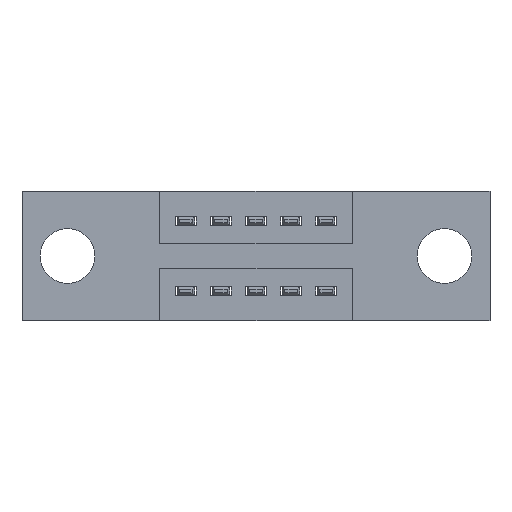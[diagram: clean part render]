
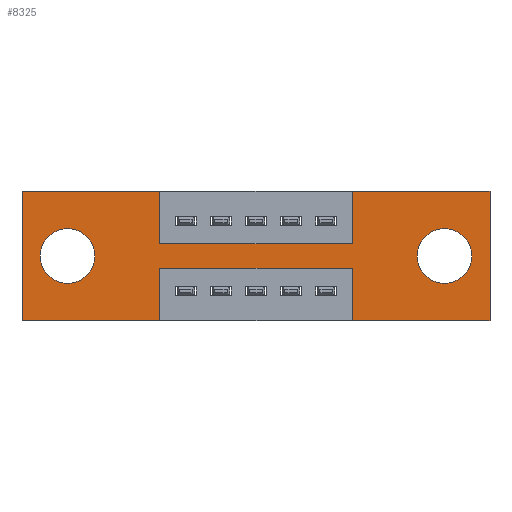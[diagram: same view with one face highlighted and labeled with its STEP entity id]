
A CAD part, front view. The second image highlights one B-rep face of the part: STEP entity #8325.
In plain terms, the highlighted planar face has unit normal (0, -1, 0).
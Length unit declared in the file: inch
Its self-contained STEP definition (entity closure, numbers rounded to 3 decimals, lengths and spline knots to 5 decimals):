
#27 = DIRECTION ( 'NONE',  ( 0., 0., -1. ) ) ;
#56 = CIRCLE ( 'NONE', #2619, 0.078 ) ;
#59 = CIRCLE ( 'NONE', #1636, 0.078 ) ;
#77 = EDGE_CURVE ( 'NONE', #8403, #8178, #6457, .T. ) ;
#88 = VECTOR ( 'NONE', #1015, 39.37008 ) ;
#94 = LINE ( 'NONE', #2735, #6843 ) ;
#206 = DIRECTION ( 'NONE',  ( 0., 0., -1. ) ) ;
#236 = EDGE_CURVE ( 'NONE', #5927, #4258, #5038, .T. ) ;
#280 = ORIENTED_EDGE ( 'NONE', *, *, #5245, .F. ) ;
#344 = EDGE_CURVE ( 'NONE', #1747, #5927, #2387, .T. ) ;
#406 = EDGE_CURVE ( 'NONE', #2341, #8580, #4386, .T. ) ;
#566 = DIRECTION ( 'NONE',  ( 0., 0., -1. ) ) ;
#583 = ORIENTED_EDGE ( 'NONE', *, *, #406, .F. ) ;
#667 = CARTESIAN_POINT ( 'NONE',  ( 0.3925, 0., -0.15 ) ) ;
#710 = PLANE ( 'NONE',  #906 ) ;
#735 = DIRECTION ( 'NONE',  ( 1., 0., 0. ) ) ;
#906 = AXIS2_PLACEMENT_3D ( 'NONE', #5362, #3974, #27 ) ;
#981 = CARTESIAN_POINT ( 'NONE',  ( 1.205, 0., -0.107 ) ) ;
#1015 = DIRECTION ( 'NONE',  ( -1., 0., 0. ) ) ;
#1120 = CARTESIAN_POINT ( 'NONE',  ( 0., 0., 0. ) ) ;
#1133 = CARTESIAN_POINT ( 'NONE',  ( 0., 0., 0. ) ) ;
#1135 = LINE ( 'NONE', #8387, #2388 ) ;
#1307 = ORIENTED_EDGE ( 'NONE', *, *, #236, .F. ) ;
#1377 = ORIENTED_EDGE ( 'NONE', *, *, #7110, .F. ) ;
#1396 = DIRECTION ( 'NONE',  ( -1., 0., 0. ) ) ;
#1445 = DIRECTION ( 'NONE',  ( 0., 1., 0. ) ) ;
#1485 = ORIENTED_EDGE ( 'NONE', *, *, #7705, .F. ) ;
#1506 = EDGE_CURVE ( 'NONE', #4596, #8403, #6110, .T. ) ;
#1546 = CARTESIAN_POINT ( 'NONE',  ( 0.3925, 0., -0.37 ) ) ;
#1636 = AXIS2_PLACEMENT_3D ( 'NONE', #3687, #2991, #3114 ) ;
#1641 = DIRECTION ( 'NONE',  ( 0., 0., 1. ) ) ;
#1666 = VERTEX_POINT ( 'NONE', #4613 ) ;
#1695 = EDGE_LOOP ( 'NONE', ( #1485, #3942, #583, #1377, #2358, #280, #1307, #4324, #3723, #8166, #3185, #7621 ) ) ;
#1747 = VERTEX_POINT ( 'NONE', #667 ) ;
#1890 = CARTESIAN_POINT ( 'NONE',  ( 0.9425, 0., 0. ) ) ;
#1973 = CARTESIAN_POINT ( 'NONE',  ( 0., 0., 0. ) ) ;
#2021 = CARTESIAN_POINT ( 'NONE',  ( 0., 0., -0.37 ) ) ;
#2030 = CARTESIAN_POINT ( 'NONE',  ( 0.9425, 0., -0.37 ) ) ;
#2341 = VERTEX_POINT ( 'NONE', #4839 ) ;
#2358 = ORIENTED_EDGE ( 'NONE', *, *, #3750, .F. ) ;
#2387 = LINE ( 'NONE', #4078, #6714 ) ;
#2388 = VECTOR ( 'NONE', #2389, 39.37008 ) ;
#2389 = DIRECTION ( 'NONE',  ( 1., 0., 0. ) ) ;
#2505 = EDGE_CURVE ( 'NONE', #8580, #6228, #8431, .T. ) ;
#2516 = VECTOR ( 'NONE', #1396, 39.37008 ) ;
#2595 = VECTOR ( 'NONE', #7276, 39.37008 ) ;
#2619 = AXIS2_PLACEMENT_3D ( 'NONE', #6319, #2947, #1641 ) ;
#2651 = ORIENTED_EDGE ( 'NONE', *, *, #5657, .T. ) ;
#2672 = ORIENTED_EDGE ( 'NONE', *, *, #6633, .T. ) ;
#2735 = CARTESIAN_POINT ( 'NONE',  ( 0., 0., -0.37 ) ) ;
#2790 = VECTOR ( 'NONE', #5843, 39.37008 ) ;
#2795 = VECTOR ( 'NONE', #5955, 39.37008 ) ;
#2869 = CARTESIAN_POINT ( 'NONE',  ( 0.3925, 0., 0. ) ) ;
#2947 = DIRECTION ( 'NONE',  ( 0., 1., 0. ) ) ;
#2991 = DIRECTION ( 'NONE',  ( 0., 1., 0. ) ) ;
#3114 = DIRECTION ( 'NONE',  ( 0., 0., -1. ) ) ;
#3185 = ORIENTED_EDGE ( 'NONE', *, *, #77, .F. ) ;
#3373 = EDGE_CURVE ( 'NONE', #8178, #3380, #1135, .T. ) ;
#3380 = VERTEX_POINT ( 'NONE', #4952 ) ;
#3415 = LINE ( 'NONE', #6698, #5333 ) ;
#3417 = DIRECTION ( 'NONE',  ( -1., 0., 0. ) ) ;
#3446 = CARTESIAN_POINT ( 'NONE',  ( 0., 0., -0.37 ) ) ;
#3641 = CARTESIAN_POINT ( 'NONE',  ( 1.335, 0., 0. ) ) ;
#3687 = CARTESIAN_POINT ( 'NONE',  ( 1.205, 0., -0.185 ) ) ;
#3723 = ORIENTED_EDGE ( 'NONE', *, *, #7919, .F. ) ;
#3750 = EDGE_CURVE ( 'NONE', #7004, #1666, #8625, .T. ) ;
#3820 = CARTESIAN_POINT ( 'NONE',  ( 0.9425, 0., -0.15 ) ) ;
#3942 = ORIENTED_EDGE ( 'NONE', *, *, #2505, .F. ) ;
#3974 = DIRECTION ( 'NONE',  ( 0., -1., 0. ) ) ;
#3983 = CARTESIAN_POINT ( 'NONE',  ( 0.9425, 0., 0. ) ) ;
#4040 = CARTESIAN_POINT ( 'NONE',  ( 1.205, 0., -0.263 ) ) ;
#4078 = CARTESIAN_POINT ( 'NONE',  ( 0.3925, 0., -0.15 ) ) ;
#4133 = VERTEX_POINT ( 'NONE', #981 ) ;
#4258 = VERTEX_POINT ( 'NONE', #1890 ) ;
#4324 = ORIENTED_EDGE ( 'NONE', *, *, #344, .F. ) ;
#4386 = LINE ( 'NONE', #2030, #2595 ) ;
#4460 = FACE_BOUND ( 'NONE', #7016, .T. ) ;
#4476 = VERTEX_POINT ( 'NONE', #7583 ) ;
#4580 = EDGE_CURVE ( 'NONE', #4476, #8059, #56, .T. ) ;
#4596 = VERTEX_POINT ( 'NONE', #1546 ) ;
#4613 = CARTESIAN_POINT ( 'NONE',  ( 1.335, 0., -0.37 ) ) ;
#4656 = CARTESIAN_POINT ( 'NONE',  ( 1.205, 0., -0.185 ) ) ;
#4667 = AXIS2_PLACEMENT_3D ( 'NONE', #7616, #1445, #6278 ) ;
#4770 = CARTESIAN_POINT ( 'NONE',  ( 0.3925, 0., -0.22 ) ) ;
#4801 = LINE ( 'NONE', #2869, #7028 ) ;
#4839 = CARTESIAN_POINT ( 'NONE',  ( 0.9425, 0., -0.37 ) ) ;
#4952 = CARTESIAN_POINT ( 'NONE',  ( 0.3925, 0., 0. ) ) ;
#5004 = FACE_OUTER_BOUND ( 'NONE', #1695, .T. ) ;
#5038 = LINE ( 'NONE', #3983, #2795 ) ;
#5148 = DIRECTION ( 'NONE',  ( 1., 0., 0. ) ) ;
#5192 = VECTOR ( 'NONE', #6219, 39.37008 ) ;
#5202 = LINE ( 'NONE', #1120, #5936 ) ;
#5245 = EDGE_CURVE ( 'NONE', #4258, #7004, #5202, .T. ) ;
#5326 = EDGE_LOOP ( 'NONE', ( #2651, #8086 ) ) ;
#5333 = VECTOR ( 'NONE', #566, 39.37008 ) ;
#5362 = CARTESIAN_POINT ( 'NONE',  ( 0., 0., -0.37 ) ) ;
#5601 = CIRCLE ( 'NONE', #8241, 0.078 ) ;
#5657 = EDGE_CURVE ( 'NONE', #8059, #4476, #8262, .T. ) ;
#5843 = DIRECTION ( 'NONE',  ( 0., 0., -1. ) ) ;
#5927 = VERTEX_POINT ( 'NONE', #3820 ) ;
#5936 = VECTOR ( 'NONE', #5148, 39.37008 ) ;
#5955 = DIRECTION ( 'NONE',  ( 0., 0., 1. ) ) ;
#6012 = DIRECTION ( 'NONE',  ( 0., 1., 0. ) ) ;
#6047 = DIRECTION ( 'NONE',  ( 0., 0., -1. ) ) ;
#6110 = LINE ( 'NONE', #3446, #2516 ) ;
#6219 = DIRECTION ( 'NONE',  ( 0., 0., 1. ) ) ;
#6228 = VERTEX_POINT ( 'NONE', #4770 ) ;
#6278 = DIRECTION ( 'NONE',  ( 0., 0., 1. ) ) ;
#6319 = CARTESIAN_POINT ( 'NONE',  ( 0.13, 0., -0.185 ) ) ;
#6457 = LINE ( 'NONE', #1973, #5192 ) ;
#6633 = EDGE_CURVE ( 'NONE', #4133, #8298, #5601, .T. ) ;
#6698 = CARTESIAN_POINT ( 'NONE',  ( 0.3925, 0., -0.37 ) ) ;
#6714 = VECTOR ( 'NONE', #735, 39.37008 ) ;
#6843 = VECTOR ( 'NONE', #3417, 39.37008 ) ;
#7004 = VERTEX_POINT ( 'NONE', #7809 ) ;
#7008 = FACE_BOUND ( 'NONE', #5326, .T. ) ;
#7016 = EDGE_LOOP ( 'NONE', ( #2672, #7431 ) ) ;
#7028 = VECTOR ( 'NONE', #206, 39.37008 ) ;
#7064 = CARTESIAN_POINT ( 'NONE',  ( 0.9425, 0., -0.22 ) ) ;
#7071 = CARTESIAN_POINT ( 'NONE',  ( 0.13, 0., -0.107 ) ) ;
#7110 = EDGE_CURVE ( 'NONE', #1666, #2341, #94, .T. ) ;
#7276 = DIRECTION ( 'NONE',  ( 0., 0., 1. ) ) ;
#7431 = ORIENTED_EDGE ( 'NONE', *, *, #8005, .T. ) ;
#7583 = CARTESIAN_POINT ( 'NONE',  ( 0.13, 0., -0.263 ) ) ;
#7616 = CARTESIAN_POINT ( 'NONE',  ( 0.13, 0., -0.185 ) ) ;
#7621 = ORIENTED_EDGE ( 'NONE', *, *, #1506, .F. ) ;
#7705 = EDGE_CURVE ( 'NONE', #6228, #4596, #3415, .T. ) ;
#7809 = CARTESIAN_POINT ( 'NONE',  ( 1.335, 0., 0. ) ) ;
#7919 = EDGE_CURVE ( 'NONE', #3380, #1747, #4801, .T. ) ;
#8005 = EDGE_CURVE ( 'NONE', #8298, #4133, #59, .T. ) ;
#8059 = VERTEX_POINT ( 'NONE', #7071 ) ;
#8086 = ORIENTED_EDGE ( 'NONE', *, *, #4580, .T. ) ;
#8166 = ORIENTED_EDGE ( 'NONE', *, *, #3373, .F. ) ;
#8178 = VERTEX_POINT ( 'NONE', #1133 ) ;
#8241 = AXIS2_PLACEMENT_3D ( 'NONE', #4656, #6012, #6047 ) ;
#8262 = CIRCLE ( 'NONE', #4667, 0.078 ) ;
#8298 = VERTEX_POINT ( 'NONE', #4040 ) ;
#8325 = ADVANCED_FACE ( 'NONE', ( #4460, #7008, #5004 ), #710, .T. ) ;
#8387 = CARTESIAN_POINT ( 'NONE',  ( 0., 0., 0. ) ) ;
#8403 = VERTEX_POINT ( 'NONE', #2021 ) ;
#8431 = LINE ( 'NONE', #8478, #88 ) ;
#8478 = CARTESIAN_POINT ( 'NONE',  ( 0.3925, 0., -0.22 ) ) ;
#8580 = VERTEX_POINT ( 'NONE', #7064 ) ;
#8625 = LINE ( 'NONE', #3641, #2790 ) ;
